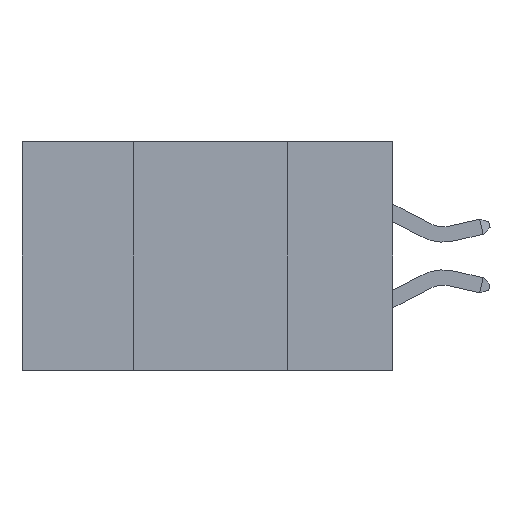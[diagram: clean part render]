
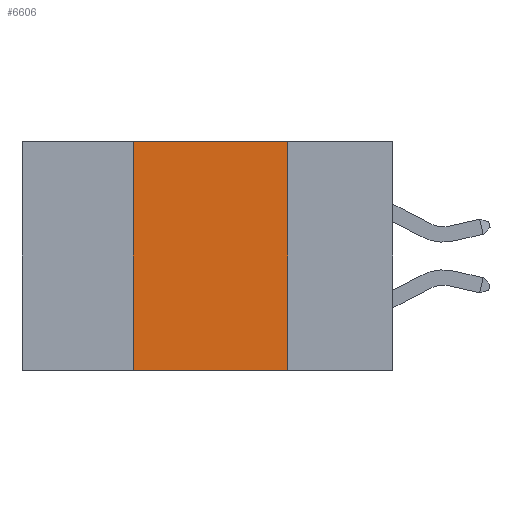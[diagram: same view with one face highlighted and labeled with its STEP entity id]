
A CAD part, left-side view. The second image highlights one B-rep face of the part: STEP entity #6606.
In plain terms, the highlighted planar face has unit normal (-1, 0, 0).
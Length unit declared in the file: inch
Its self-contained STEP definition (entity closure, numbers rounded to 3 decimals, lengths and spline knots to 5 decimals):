
#628 = CARTESIAN_POINT ( 'NONE',  ( 0., 0.17, -0.37 ) ) ;
#690 = EDGE_CURVE ( 'NONE', #808, #5430, #3232, .T. ) ;
#808 = VERTEX_POINT ( 'NONE', #2506 ) ;
#1392 = CARTESIAN_POINT ( 'NONE',  ( 0., 0.17, 0. ) ) ;
#1662 = CARTESIAN_POINT ( 'NONE',  ( 0., 0.6, 0. ) ) ;
#2034 = ORIENTED_EDGE ( 'NONE', *, *, #3677, .F. ) ;
#2093 = AXIS2_PLACEMENT_3D ( 'NONE', #6418, #9806, #8968 ) ;
#2189 = VERTEX_POINT ( 'NONE', #1392 ) ;
#2506 = CARTESIAN_POINT ( 'NONE',  ( 0., 0.42, -0.37 ) ) ;
#2567 = EDGE_CURVE ( 'NONE', #808, #5047, #8114, .T. ) ;
#2809 = VECTOR ( 'NONE', #4225, 39.37008 ) ;
#3232 = LINE ( 'NONE', #3288, #8302 ) ;
#3288 = CARTESIAN_POINT ( 'NONE',  ( 0., 0.6, -0.37 ) ) ;
#3577 = VECTOR ( 'NONE', #8277, 39.37008 ) ;
#3677 = EDGE_CURVE ( 'NONE', #2189, #5430, #10181, .T. ) ;
#4225 = DIRECTION ( 'NONE',  ( 0., -1., 0. ) ) ;
#4229 = DIRECTION ( 'NONE',  ( 0., 0., -1. ) ) ;
#5047 = VERTEX_POINT ( 'NONE', #7697 ) ;
#5430 = VERTEX_POINT ( 'NONE', #628 ) ;
#5547 = EDGE_CURVE ( 'NONE', #5047, #2189, #9282, .T. ) ;
#5894 = CARTESIAN_POINT ( 'NONE',  ( 0., 0.17, 0. ) ) ;
#6282 = ORIENTED_EDGE ( 'NONE', *, *, #690, .T. ) ;
#6418 = CARTESIAN_POINT ( 'NONE',  ( 0., 0.6, 0. ) ) ;
#6606 = ADVANCED_FACE ( 'NONE', ( #10586 ), #10477, .F. ) ;
#6686 = DIRECTION ( 'NONE',  ( 0., -1., 0. ) ) ;
#6692 = EDGE_LOOP ( 'NONE', ( #2034, #7103, #8122, #6282 ) ) ;
#7103 = ORIENTED_EDGE ( 'NONE', *, *, #5547, .F. ) ;
#7557 = VECTOR ( 'NONE', #4229, 39.37008 ) ;
#7697 = CARTESIAN_POINT ( 'NONE',  ( 0., 0.42, 0. ) ) ;
#8114 = LINE ( 'NONE', #9828, #3577 ) ;
#8122 = ORIENTED_EDGE ( 'NONE', *, *, #2567, .F. ) ;
#8277 = DIRECTION ( 'NONE',  ( 0., 0., 1. ) ) ;
#8302 = VECTOR ( 'NONE', #6686, 39.37008 ) ;
#8968 = DIRECTION ( 'NONE',  ( 0., 0., -1. ) ) ;
#9282 = LINE ( 'NONE', #1662, #2809 ) ;
#9806 = DIRECTION ( 'NONE',  ( 1., 0., 0. ) ) ;
#9828 = CARTESIAN_POINT ( 'NONE',  ( 0., 0.42, 0. ) ) ;
#10181 = LINE ( 'NONE', #5894, #7557 ) ;
#10477 = PLANE ( 'NONE',  #2093 ) ;
#10586 = FACE_OUTER_BOUND ( 'NONE', #6692, .T. ) ;
